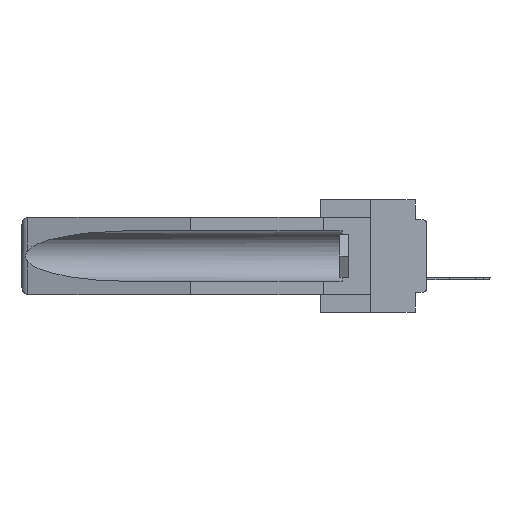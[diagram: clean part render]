
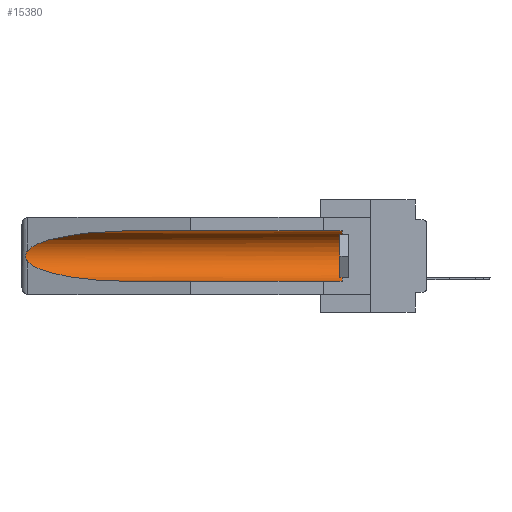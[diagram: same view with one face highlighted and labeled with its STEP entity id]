
A CAD part, left-side view. The second image highlights one B-rep face of the part: STEP entity #15380.
In plain terms, the highlighted cylindrical face has radius 2.857 mm (diameter 5.715 mm), a partial arc.
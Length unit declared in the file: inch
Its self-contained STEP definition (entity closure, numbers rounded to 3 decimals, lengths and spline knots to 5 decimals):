
#135 = CARTESIAN_POINT ( 'NONE',  ( 0.155, -0.30754, -0.059 ) ) ;
#218 = CARTESIAN_POINT ( 'NONE',  ( 0.26597, 1.5296, -0.19026 ) ) ;
#676 = CARTESIAN_POINT ( 'NONE',  ( 0.26537, 1.52718, -0.14972 ) ) ;
#738 = DIRECTION ( 'NONE',  ( 0., -1., 0. ) ) ;
#1437 = CARTESIAN_POINT ( 'NONE',  ( 0.155, -0.30754, -0.284 ) ) ;
#1692 = FACE_OUTER_BOUND ( 'NONE', #24928, .T. ) ;
#1731 = ORIENTED_EDGE ( 'NONE', *, *, #2263, .T. ) ;
#2263 = EDGE_CURVE ( 'NONE', #10742, #17760, #14753, .T. ) ;
#3403 = AXIS2_PLACEMENT_3D ( 'NONE', #20406, #13341, #23078 ) ;
#3735 = ORIENTED_EDGE ( 'NONE', *, *, #12165, .T. ) ;
#4792 = CARTESIAN_POINT ( 'NONE',  ( 0.155, 0.126, -0.059 ) ) ;
#5329 = DIRECTION ( 'NONE',  ( 0., 1., 0. ) ) ;
#7298 = CIRCLE ( 'NONE', #26898, 0.1125 ) ;
#8387 = CARTESIAN_POINT ( 'NONE',  ( 0.26537, 1.52718, -0.19328 ) ) ;
#10281 = CARTESIAN_POINT ( 'NONE',  ( 0.2675, 1.53308, -0.16763 ) ) ;
#10345 = DIRECTION ( 'NONE',  ( 0., 0., 1. ) ) ;
#10599 = CARTESIAN_POINT ( 'NONE',  ( 0.21114, 1.30732, -0.284 ) ) ;
#10661 = ORIENTED_EDGE ( 'NONE', *, *, #23200, .F. ) ;
#10703 = VERTEX_POINT ( 'NONE', #23494 ) ;
#10742 = VERTEX_POINT ( 'NONE', #4792 ) ;
#10812 = EDGE_CURVE ( 'NONE', #10703, #25004, #27206, .T. ) ;
#10996 = EDGE_CURVE ( 'NONE', #25004, #24932, #25573, .T. ) ;
#11171 = DIRECTION ( 'NONE',  ( 0., 1., 0. ) ) ;
#11827 = CARTESIAN_POINT ( 'NONE',  ( 0.155, 0.126, -0.284 ) ) ;
#12015 = CARTESIAN_POINT ( 'NONE',  ( 0.26654, 1.53092, -0.15636 ) ) ;
#12165 = EDGE_CURVE ( 'NONE', #17760, #10703, #26354, .T. ) ;
#12172 = CARTESIAN_POINT ( 'NONE',  ( 0.26655, 1.53094, -0.18657 ) ) ;
#12705 = CARTESIAN_POINT ( 'NONE',  ( 0.155, 0.126, -0.1715 ) ) ;
#13341 = DIRECTION ( 'NONE',  ( 0., 1., 0. ) ) ;
#13379 = ORIENTED_EDGE ( 'NONE', *, *, #10996, .T. ) ;
#13645 = CYLINDRICAL_SURFACE ( 'NONE', #3403, 0.1125 ) ;
#14753 = LINE ( 'NONE', #135, #29647 ) ;
#15145 = CARTESIAN_POINT ( 'NONE',  ( 0.26537, 1.52718, -0.19328 ) ) ;
#15305 = CARTESIAN_POINT ( 'NONE',  ( 0.25451, 1.48313, -0.24835 ) ) ;
#15380 = ADVANCED_FACE ( 'NONE', ( #1692 ), #13645, .F. ) ;
#15489 = CARTESIAN_POINT ( 'NONE',  ( 0.155, 1.07973, -0.059 ) ) ;
#17715 = CARTESIAN_POINT ( 'NONE',  ( 0.25451, 1.48313, -0.09465 ) ) ;
#17760 = VERTEX_POINT ( 'NONE', #27051 ) ;
#20406 = CARTESIAN_POINT ( 'NONE',  ( 0.155, -0.30754, -0.1715 ) ) ;
#20504 = CARTESIAN_POINT ( 'NONE',  ( 0.21114, 1.30732, -0.059 ) ) ;
#20611 = LINE ( 'NONE', #1437, #28197 ) ;
#21765 = CARTESIAN_POINT ( 'NONE',  ( 0.26597, 1.52961, -0.15275 ) ) ;
#21917 = CARTESIAN_POINT ( 'NONE',  ( 0.2673, 1.53269, -0.17917 ) ) ;
#22387 = CARTESIAN_POINT ( 'NONE',  ( 0.155, 1.07973, -0.284 ) ) ;
#22388 = CARTESIAN_POINT ( 'NONE',  ( 0.26537, 1.52718, -0.19328 ) ) ;
#23078 = DIRECTION ( 'NONE',  ( 0., 0., 1. ) ) ;
#23200 = EDGE_CURVE ( 'NONE', #26559, #24932, #20611, .T. ) ;
#23494 = CARTESIAN_POINT ( 'NONE',  ( 0.26537, 1.52718, -0.14972 ) ) ;
#23810 = CARTESIAN_POINT ( 'NONE',  ( 0.155, 1.07973, -0.284 ) ) ;
#24438 = ORIENTED_EDGE ( 'NONE', *, *, #28545, .T. ) ;
#24928 = EDGE_LOOP ( 'NONE', ( #3735, #30589, #13379, #10661, #24438, #1731 ) ) ;
#24932 = VERTEX_POINT ( 'NONE', #23810 ) ;
#25004 = VERTEX_POINT ( 'NONE', #22388 ) ;
#25573 =( BOUNDED_CURVE ( )  B_SPLINE_CURVE ( 3, ( #8387, #15305, #10599, #22387 ),
 .UNSPECIFIED., .F., .F. ) 
 B_SPLINE_CURVE_WITH_KNOTS ( ( 4, 4 ),
 ( 0.1948, 1.5708 ),
 .UNSPECIFIED. ) 
 CURVE ( )  GEOMETRIC_REPRESENTATION_ITEM ( )  RATIONAL_B_SPLINE_CURVE ( ( 1., 0.848, 0.848, 1. ) ) 
 REPRESENTATION_ITEM ( '' )  );
#26354 =( BOUNDED_CURVE ( )  B_SPLINE_CURVE ( 3, ( #15489, #20504, #17715, #27745 ),
 .UNSPECIFIED., .F., .F. ) 
 B_SPLINE_CURVE_WITH_KNOTS ( ( 4, 4 ),
 ( 4.71239, 6.08839 ),
 .UNSPECIFIED. ) 
 CURVE ( )  GEOMETRIC_REPRESENTATION_ITEM ( )  RATIONAL_B_SPLINE_CURVE ( ( 1., 0.848, 0.848, 1. ) ) 
 REPRESENTATION_ITEM ( '' )  );
#26559 = VERTEX_POINT ( 'NONE', #11827 ) ;
#26898 = AXIS2_PLACEMENT_3D ( 'NONE', #12705, #738, #10345 ) ;
#27051 = CARTESIAN_POINT ( 'NONE',  ( 0.155, 1.07973, -0.059 ) ) ;
#27206 = B_SPLINE_CURVE_WITH_KNOTS ( 'NONE', 3,
 ( #676, #21765, #12015, #29465, #10281, #29167, #21917, #12172, #218, #15145 ),
 .UNSPECIFIED., .F., .F.,
 ( 4, 2, 2, 2, 4 ),
 ( 0., 0.00029, 0.00058, 0.00087, 0.00117 ),
 .UNSPECIFIED. ) ;
#27745 = CARTESIAN_POINT ( 'NONE',  ( 0.26537, 1.52718, -0.14972 ) ) ;
#28197 = VECTOR ( 'NONE', #11171, 39.37008 ) ;
#28545 = EDGE_CURVE ( 'NONE', #26559, #10742, #7298, .T. ) ;
#29167 = CARTESIAN_POINT ( 'NONE',  ( 0.2675, 1.53308, -0.17534 ) ) ;
#29465 = CARTESIAN_POINT ( 'NONE',  ( 0.2673, 1.5327, -0.16383 ) ) ;
#29647 = VECTOR ( 'NONE', #5329, 39.37008 ) ;
#30589 = ORIENTED_EDGE ( 'NONE', *, *, #10812, .T. ) ;
